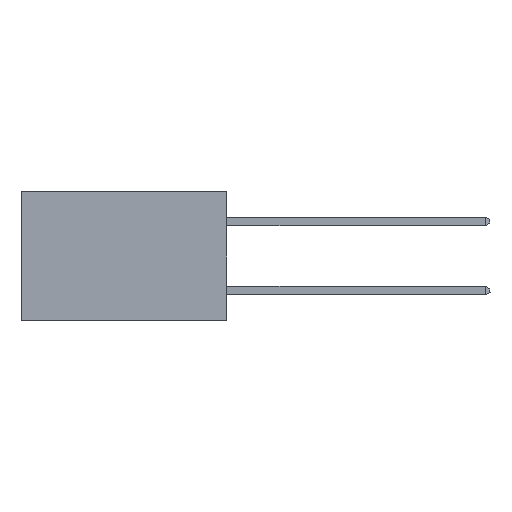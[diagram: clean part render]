
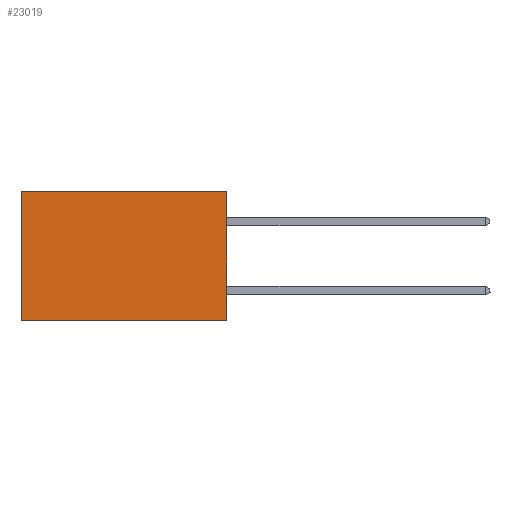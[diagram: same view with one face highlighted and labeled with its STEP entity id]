
A CAD part, left-side view. The second image highlights one B-rep face of the part: STEP entity #23019.
In plain terms, the highlighted planar face has unit normal (-1, 0, 0).
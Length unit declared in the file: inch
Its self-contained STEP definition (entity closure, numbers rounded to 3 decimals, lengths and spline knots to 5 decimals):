
#588 = AXIS2_PLACEMENT_3D ( 'NONE', #12472, #3179, #16151 ) ;
#1295 = CARTESIAN_POINT ( 'NONE',  ( 0.277, 0., -0.37 ) ) ;
#1744 = VECTOR ( 'NONE', #7331, 39.37008 ) ;
#1822 = ORIENTED_EDGE ( 'NONE', *, *, #17181, .T. ) ;
#1926 = VERTEX_POINT ( 'NONE', #22391 ) ;
#2063 = VECTOR ( 'NONE', #19874, 39.37008 ) ;
#2432 = EDGE_CURVE ( 'NONE', #9581, #7370, #11661, .T. ) ;
#3062 = VERTEX_POINT ( 'NONE', #15641 ) ;
#3179 = DIRECTION ( 'NONE',  ( 1., 0., 0. ) ) ;
#3271 = VECTOR ( 'NONE', #3816, 39.37008 ) ;
#3816 = DIRECTION ( 'NONE',  ( 0., 1., 0. ) ) ;
#3844 = LINE ( 'NONE', #4158, #3271 ) ;
#4158 = CARTESIAN_POINT ( 'NONE',  ( 0.277, 0., 0. ) ) ;
#7143 = EDGE_CURVE ( 'NONE', #9581, #1926, #3844, .T. ) ;
#7331 = DIRECTION ( 'NONE',  ( 0., 0., -1. ) ) ;
#7370 = VERTEX_POINT ( 'NONE', #1295 ) ;
#7619 = CARTESIAN_POINT ( 'NONE',  ( 0.277, 0., 0. ) ) ;
#9327 = LINE ( 'NONE', #20600, #23374 ) ;
#9581 = VERTEX_POINT ( 'NONE', #7619 ) ;
#9624 = DIRECTION ( 'NONE',  ( 0., 0., -1. ) ) ;
#10090 = ORIENTED_EDGE ( 'NONE', *, *, #2432, .F. ) ;
#11661 = LINE ( 'NONE', #18610, #1744 ) ;
#12472 = CARTESIAN_POINT ( 'NONE',  ( 0.277, 0., -0.37 ) ) ;
#14348 = CARTESIAN_POINT ( 'NONE',  ( 0.277, 0., -0.37 ) ) ;
#14416 = EDGE_CURVE ( 'NONE', #7370, #3062, #16828, .T. ) ;
#15641 = CARTESIAN_POINT ( 'NONE',  ( 0.277, 0.59, -0.37 ) ) ;
#16151 = DIRECTION ( 'NONE',  ( 0., 0., -1. ) ) ;
#16409 = EDGE_LOOP ( 'NONE', ( #1822, #18781, #10090, #16724 ) ) ;
#16724 = ORIENTED_EDGE ( 'NONE', *, *, #7143, .T. ) ;
#16828 = LINE ( 'NONE', #14348, #2063 ) ;
#17181 = EDGE_CURVE ( 'NONE', #1926, #3062, #9327, .T. ) ;
#17901 = PLANE ( 'NONE',  #588 ) ;
#18610 = CARTESIAN_POINT ( 'NONE',  ( 0.277, 0., -0.37 ) ) ;
#18781 = ORIENTED_EDGE ( 'NONE', *, *, #14416, .F. ) ;
#19874 = DIRECTION ( 'NONE',  ( 0., 1., 0. ) ) ;
#20600 = CARTESIAN_POINT ( 'NONE',  ( 0.277, 0.59, -0.37 ) ) ;
#21177 = FACE_OUTER_BOUND ( 'NONE', #16409, .T. ) ;
#22391 = CARTESIAN_POINT ( 'NONE',  ( 0.277, 0.59, 0. ) ) ;
#23019 = ADVANCED_FACE ( 'NONE', ( #21177 ), #17901, .F. ) ;
#23374 = VECTOR ( 'NONE', #9624, 39.37008 ) ;
